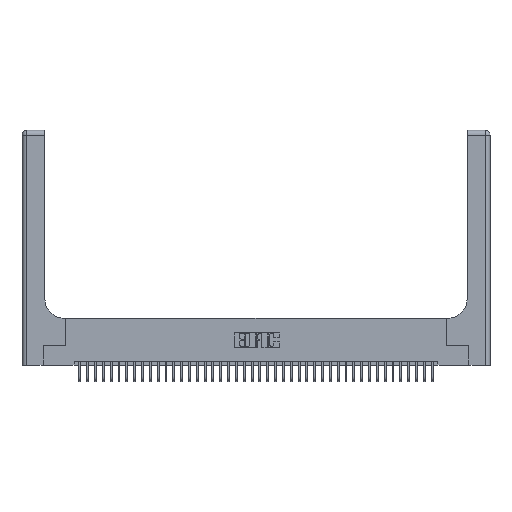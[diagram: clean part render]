
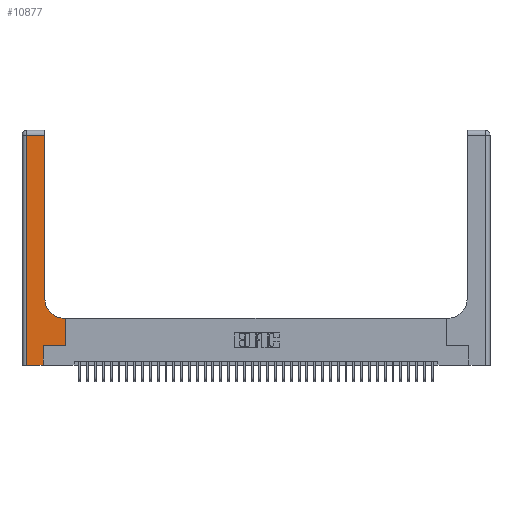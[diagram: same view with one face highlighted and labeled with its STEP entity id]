
A CAD part, top view. The second image highlights one B-rep face of the part: STEP entity #10877.
In plain terms, the highlighted planar face has unit normal (0, 0, 1).
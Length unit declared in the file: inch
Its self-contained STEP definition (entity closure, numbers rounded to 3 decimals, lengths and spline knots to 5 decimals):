
#137 = ORIENTED_EDGE ( 'NONE', *, *, #33319, .T. ) ;
#455 = EDGE_CURVE ( 'NONE', #25529, #8511, #10581, .T. ) ;
#640 = VECTOR ( 'NONE', #11815, 39.37008 ) ;
#1005 = DIRECTION ( 'NONE',  ( -1., 0., 0. ) ) ;
#1946 = EDGE_LOOP ( 'NONE', ( #30744, #26772, #37737, #9559, #37973, #137, #27083, #19459, #9896 ) ) ;
#2130 = CARTESIAN_POINT ( 'NONE',  ( 0.06, 3., 0.37 ) ) ;
#2437 = VERTEX_POINT ( 'NONE', #32477 ) ;
#2590 = DIRECTION ( 'NONE',  ( 0., 0., -1. ) ) ;
#3100 = PLANE ( 'NONE',  #10118 ) ;
#3734 = EDGE_CURVE ( 'NONE', #4808, #20826, #33452, .T. ) ;
#3981 = CARTESIAN_POINT ( 'NONE',  ( 0.06, 2.94, 0.37 ) ) ;
#4367 = VERTEX_POINT ( 'NONE', #28319 ) ;
#4808 = VERTEX_POINT ( 'NONE', #14573 ) ;
#6625 = LINE ( 'NONE', #28314, #28580 ) ;
#8511 = VERTEX_POINT ( 'NONE', #3981 ) ;
#9559 = ORIENTED_EDGE ( 'NONE', *, *, #9640, .T. ) ;
#9563 = VECTOR ( 'NONE', #1005, 39.37008 ) ;
#9640 = EDGE_CURVE ( 'NONE', #4367, #31495, #12998, .T. ) ;
#9835 = LINE ( 'NONE', #2130, #35983 ) ;
#9896 = ORIENTED_EDGE ( 'NONE', *, *, #3734, .T. ) ;
#10005 = EDGE_CURVE ( 'NONE', #37484, #4808, #10401, .T. ) ;
#10118 = AXIS2_PLACEMENT_3D ( 'NONE', #22691, #16266, #39194 ) ;
#10401 = LINE ( 'NONE', #41690, #26737 ) ;
#10581 = LINE ( 'NONE', #14055, #9563 ) ;
#10669 = EDGE_CURVE ( 'NONE', #8511, #4367, #9835, .T. ) ;
#10862 = VECTOR ( 'NONE', #22532, 39.37008 ) ;
#10877 = ADVANCED_FACE ( 'NONE', ( #30806 ), #3100, .F. ) ;
#11815 = DIRECTION ( 'NONE',  ( 0., 1., 0. ) ) ;
#11875 = LINE ( 'NONE', #25693, #10862 ) ;
#12998 = LINE ( 'NONE', #20635, #38120 ) ;
#13155 = EDGE_CURVE ( 'NONE', #31495, #2437, #22372, .T. ) ;
#14055 = CARTESIAN_POINT ( 'NONE',  ( 0., 2.94, 0.37 ) ) ;
#14573 = CARTESIAN_POINT ( 'NONE',  ( 0.5415, 0.6, 0.37 ) ) ;
#15303 = DIRECTION ( 'NONE',  ( 0., 1., 0. ) ) ;
#16266 = DIRECTION ( 'NONE',  ( 0., 0., -1. ) ) ;
#17351 = DIRECTION ( 'NONE',  ( 1., 0., 0. ) ) ;
#18614 = DIRECTION ( 'NONE',  ( -1., 0., 0. ) ) ;
#19459 = ORIENTED_EDGE ( 'NONE', *, *, #10005, .T. ) ;
#19618 = CARTESIAN_POINT ( 'NONE',  ( 0.269, 0., 0.37 ) ) ;
#19754 = DIRECTION ( 'NONE',  ( 0., 1., 0. ) ) ;
#20089 = LINE ( 'NONE', #28104, #640 ) ;
#20635 = CARTESIAN_POINT ( 'NONE',  ( 0., 0., 0.37 ) ) ;
#20657 = AXIS2_PLACEMENT_3D ( 'NONE', #22185, #2590, #25461 ) ;
#20826 = VERTEX_POINT ( 'NONE', #37776 ) ;
#22185 = CARTESIAN_POINT ( 'NONE',  ( 0.5415, 0.85, 0.37 ) ) ;
#22372 = LINE ( 'NONE', #19618, #30073 ) ;
#22532 = DIRECTION ( 'NONE',  ( 1., 0., 0. ) ) ;
#22691 = CARTESIAN_POINT ( 'NONE',  ( 0., 3., 0.37 ) ) ;
#24987 = DIRECTION ( 'NONE',  ( 0., -1., 0. ) ) ;
#25461 = DIRECTION ( 'NONE',  ( 1., 0., 0. ) ) ;
#25529 = VERTEX_POINT ( 'NONE', #28307 ) ;
#25693 = CARTESIAN_POINT ( 'NONE',  ( 0.269, 0.25, 0.37 ) ) ;
#26736 = CARTESIAN_POINT ( 'NONE',  ( 0.5585, 0.25, 0.37 ) ) ;
#26737 = VECTOR ( 'NONE', #18614, 39.37008 ) ;
#26772 = ORIENTED_EDGE ( 'NONE', *, *, #455, .T. ) ;
#27083 = ORIENTED_EDGE ( 'NONE', *, *, #33120, .T. ) ;
#28104 = CARTESIAN_POINT ( 'NONE',  ( 0.5585, 0.25, 0.37 ) ) ;
#28307 = CARTESIAN_POINT ( 'NONE',  ( 0.2915, 2.94, 0.37 ) ) ;
#28314 = CARTESIAN_POINT ( 'NONE',  ( 0.2915, 3., 0.37 ) ) ;
#28319 = CARTESIAN_POINT ( 'NONE',  ( 0.06, 0., 0.37 ) ) ;
#28580 = VECTOR ( 'NONE', #15303, 39.37008 ) ;
#29405 = CARTESIAN_POINT ( 'NONE',  ( 0.269, 0., 0.37 ) ) ;
#29418 = CARTESIAN_POINT ( 'NONE',  ( 0.5585, 0.6, 0.37 ) ) ;
#30073 = VECTOR ( 'NONE', #19754, 39.37008 ) ;
#30744 = ORIENTED_EDGE ( 'NONE', *, *, #38511, .T. ) ;
#30806 = FACE_OUTER_BOUND ( 'NONE', #1946, .T. ) ;
#31495 = VERTEX_POINT ( 'NONE', #29405 ) ;
#32477 = CARTESIAN_POINT ( 'NONE',  ( 0.269, 0.25, 0.37 ) ) ;
#33120 = EDGE_CURVE ( 'NONE', #38233, #37484, #20089, .T. ) ;
#33319 = EDGE_CURVE ( 'NONE', #2437, #38233, #11875, .T. ) ;
#33452 = CIRCLE ( 'NONE', #20657, 0.25 ) ;
#35983 = VECTOR ( 'NONE', #24987, 39.37008 ) ;
#37484 = VERTEX_POINT ( 'NONE', #29418 ) ;
#37737 = ORIENTED_EDGE ( 'NONE', *, *, #10669, .T. ) ;
#37776 = CARTESIAN_POINT ( 'NONE',  ( 0.2915, 0.85, 0.37 ) ) ;
#37973 = ORIENTED_EDGE ( 'NONE', *, *, #13155, .T. ) ;
#38120 = VECTOR ( 'NONE', #17351, 39.37008 ) ;
#38233 = VERTEX_POINT ( 'NONE', #26736 ) ;
#38511 = EDGE_CURVE ( 'NONE', #20826, #25529, #6625, .T. ) ;
#39194 = DIRECTION ( 'NONE',  ( -1., 0., 0. ) ) ;
#41690 = CARTESIAN_POINT ( 'NONE',  ( 0.2915, 0.6, 0.37 ) ) ;
